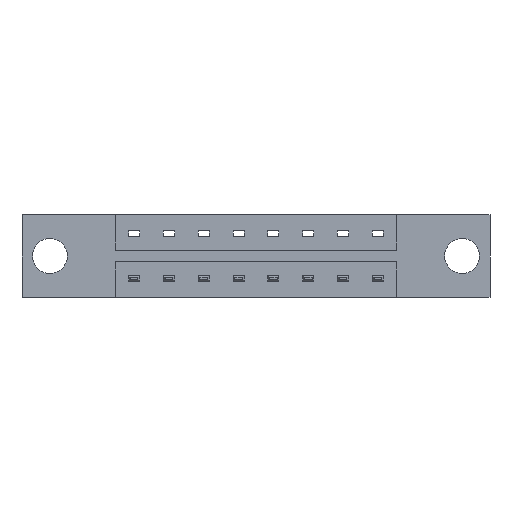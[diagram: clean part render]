
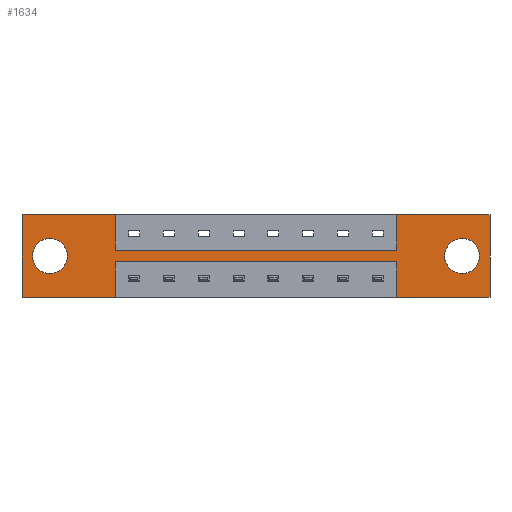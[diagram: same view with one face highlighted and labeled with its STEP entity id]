
A CAD part, front view. The second image highlights one B-rep face of the part: STEP entity #1634.
In plain terms, the highlighted planar face has unit normal (0, -1, 0).
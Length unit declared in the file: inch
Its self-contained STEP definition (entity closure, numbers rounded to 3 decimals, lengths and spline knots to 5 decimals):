
#97 = DIRECTION ( 'NONE',  ( 0., 0., -1. ) ) ;
#120 = PLANE ( 'NONE',  #6960 ) ;
#161 = ORIENTED_EDGE ( 'NONE', *, *, #1057, .F. ) ;
#222 = VERTEX_POINT ( 'NONE', #7036 ) ;
#249 = DIRECTION ( 'NONE',  ( 0., 1., 0. ) ) ;
#284 = DIRECTION ( 'NONE',  ( 0., 0., -1. ) ) ;
#331 = LINE ( 'NONE', #5976, #1162 ) ;
#354 = ORIENTED_EDGE ( 'NONE', *, *, #995, .F. ) ;
#361 = VECTOR ( 'NONE', #808, 39.37008 ) ;
#465 = CARTESIAN_POINT ( 'NONE',  ( 1.6785, 0., -0.2115 ) ) ;
#496 = EDGE_CURVE ( 'NONE', #8534, #3127, #938, .T. ) ;
#721 = VECTOR ( 'NONE', #1155, 39.37008 ) ;
#799 = VERTEX_POINT ( 'NONE', #5838 ) ;
#808 = DIRECTION ( 'NONE',  ( 0., 0., 1. ) ) ;
#862 = CARTESIAN_POINT ( 'NONE',  ( 2.096, 0., -0.37 ) ) ;
#866 = AXIS2_PLACEMENT_3D ( 'NONE', #2997, #7089, #2206 ) ;
#911 = FACE_OUTER_BOUND ( 'NONE', #1650, .T. ) ;
#921 = EDGE_CURVE ( 'NONE', #3524, #3013, #331, .T. ) ;
#938 = CIRCLE ( 'NONE', #2129, 0.078 ) ;
#964 = EDGE_LOOP ( 'NONE', ( #5237, #8915 ) ) ;
#995 = EDGE_CURVE ( 'NONE', #3325, #8049, #7485, .T. ) ;
#1000 = CARTESIAN_POINT ( 'NONE',  ( 1.6785, 0., -0.1585 ) ) ;
#1041 = CARTESIAN_POINT ( 'NONE',  ( 2.096, 0., 0. ) ) ;
#1057 = EDGE_CURVE ( 'NONE', #5483, #3524, #5420, .T. ) ;
#1097 = CARTESIAN_POINT ( 'NONE',  ( 0., 0., -0.37 ) ) ;
#1155 = DIRECTION ( 'NONE',  ( 0., 0., 1. ) ) ;
#1162 = VECTOR ( 'NONE', #284, 39.37008 ) ;
#1167 = ORIENTED_EDGE ( 'NONE', *, *, #3493, .F. ) ;
#1338 = LINE ( 'NONE', #5687, #8081 ) ;
#1478 = DIRECTION ( 'NONE',  ( -1., 0., 0. ) ) ;
#1533 = ORIENTED_EDGE ( 'NONE', *, *, #921, .F. ) ;
#1634 = ADVANCED_FACE ( 'NONE', ( #3048, #4310, #911 ), #120, .T. ) ;
#1635 = ORIENTED_EDGE ( 'NONE', *, *, #7399, .F. ) ;
#1650 = EDGE_LOOP ( 'NONE', ( #7386, #1805, #1533, #161, #2510, #6017, #1635, #354, #1167, #4787, #2770, #2639 ) ) ;
#1805 = ORIENTED_EDGE ( 'NONE', *, *, #3112, .F. ) ;
#1892 = VERTEX_POINT ( 'NONE', #5959 ) ;
#1901 = CARTESIAN_POINT ( 'NONE',  ( 0., 0., 0. ) ) ;
#2051 = CIRCLE ( 'NONE', #8232, 0.078 ) ;
#2129 = AXIS2_PLACEMENT_3D ( 'NONE', #6581, #249, #5895 ) ;
#2147 = EDGE_CURVE ( 'NONE', #3127, #8534, #3242, .T. ) ;
#2165 = VERTEX_POINT ( 'NONE', #4490 ) ;
#2206 = DIRECTION ( 'NONE',  ( 0., 0., 1. ) ) ;
#2250 = VERTEX_POINT ( 'NONE', #2610 ) ;
#2271 = DIRECTION ( 'NONE',  ( 0., 0., 1. ) ) ;
#2290 = DIRECTION ( 'NONE',  ( 0., 0., -1. ) ) ;
#2328 = VERTEX_POINT ( 'NONE', #4743 ) ;
#2404 = DIRECTION ( 'NONE',  ( 0., 0., -1. ) ) ;
#2406 = LINE ( 'NONE', #1000, #3681 ) ;
#2451 = LINE ( 'NONE', #5993, #9018 ) ;
#2510 = ORIENTED_EDGE ( 'NONE', *, *, #2916, .F. ) ;
#2610 = CARTESIAN_POINT ( 'NONE',  ( 1.6785, 0., -0.2115 ) ) ;
#2639 = ORIENTED_EDGE ( 'NONE', *, *, #4357, .F. ) ;
#2647 = VECTOR ( 'NONE', #8945, 39.37008 ) ;
#2770 = ORIENTED_EDGE ( 'NONE', *, *, #8570, .F. ) ;
#2815 = CARTESIAN_POINT ( 'NONE',  ( 0., 0., 0. ) ) ;
#2844 = AXIS2_PLACEMENT_3D ( 'NONE', #7637, #5534, #4193 ) ;
#2880 = EDGE_CURVE ( 'NONE', #2165, #799, #1338, .T. ) ;
#2916 = EDGE_CURVE ( 'NONE', #222, #5483, #2406, .T. ) ;
#2921 = EDGE_CURVE ( 'NONE', #5778, #1892, #2051, .T. ) ;
#2997 = CARTESIAN_POINT ( 'NONE',  ( 0.125, 0., -0.185 ) ) ;
#3013 = VERTEX_POINT ( 'NONE', #862 ) ;
#3048 = FACE_BOUND ( 'NONE', #4469, .T. ) ;
#3049 = DIRECTION ( 'NONE',  ( 0., 0., -1. ) ) ;
#3088 = DIRECTION ( 'NONE',  ( -1., 0., 0. ) ) ;
#3112 = EDGE_CURVE ( 'NONE', #3013, #8420, #3332, .T. ) ;
#3127 = VERTEX_POINT ( 'NONE', #3890 ) ;
#3242 = CIRCLE ( 'NONE', #866, 0.078 ) ;
#3279 = VECTOR ( 'NONE', #4741, 39.37008 ) ;
#3325 = VERTEX_POINT ( 'NONE', #2815 ) ;
#3332 = LINE ( 'NONE', #1097, #2647 ) ;
#3493 = EDGE_CURVE ( 'NONE', #799, #3325, #8708, .T. ) ;
#3524 = VERTEX_POINT ( 'NONE', #1041 ) ;
#3681 = VECTOR ( 'NONE', #2271, 39.37008 ) ;
#3714 = EDGE_CURVE ( 'NONE', #1892, #5778, #8430, .T. ) ;
#3810 = ORIENTED_EDGE ( 'NONE', *, *, #3714, .T. ) ;
#3843 = DIRECTION ( 'NONE',  ( 0., 1., 0. ) ) ;
#3890 = CARTESIAN_POINT ( 'NONE',  ( 0.125, 0., -0.107 ) ) ;
#4193 = DIRECTION ( 'NONE',  ( 0., 0., -1. ) ) ;
#4310 = FACE_BOUND ( 'NONE', #964, .T. ) ;
#4357 = EDGE_CURVE ( 'NONE', #2250, #7164, #2451, .T. ) ;
#4469 = EDGE_LOOP ( 'NONE', ( #3810, #5562 ) ) ;
#4490 = CARTESIAN_POINT ( 'NONE',  ( 0.4175, 0., -0.37 ) ) ;
#4614 = CARTESIAN_POINT ( 'NONE',  ( 0.4175, 0., -0.2115 ) ) ;
#4714 = EDGE_CURVE ( 'NONE', #2328, #222, #6488, .T. ) ;
#4741 = DIRECTION ( 'NONE',  ( 1., 0., 0. ) ) ;
#4743 = CARTESIAN_POINT ( 'NONE',  ( 0.4175, 0., -0.1585 ) ) ;
#4787 = ORIENTED_EDGE ( 'NONE', *, *, #2880, .F. ) ;
#4855 = VECTOR ( 'NONE', #8514, 39.37008 ) ;
#4871 = VECTOR ( 'NONE', #97, 39.37008 ) ;
#5237 = ORIENTED_EDGE ( 'NONE', *, *, #2147, .T. ) ;
#5420 = LINE ( 'NONE', #1901, #3279 ) ;
#5476 = VECTOR ( 'NONE', #2290, 39.37008 ) ;
#5483 = VERTEX_POINT ( 'NONE', #6736 ) ;
#5534 = DIRECTION ( 'NONE',  ( 0., 1., 0. ) ) ;
#5562 = ORIENTED_EDGE ( 'NONE', *, *, #2921, .T. ) ;
#5669 = CARTESIAN_POINT ( 'NONE',  ( 0.4175, 0., -0.1585 ) ) ;
#5687 = CARTESIAN_POINT ( 'NONE',  ( 0., 0., -0.37 ) ) ;
#5774 = DIRECTION ( 'NONE',  ( 0., -1., 0. ) ) ;
#5778 = VERTEX_POINT ( 'NONE', #6904 ) ;
#5838 = CARTESIAN_POINT ( 'NONE',  ( 0., 0., -0.37 ) ) ;
#5883 = LINE ( 'NONE', #4614, #5476 ) ;
#5895 = DIRECTION ( 'NONE',  ( 0., 0., 1. ) ) ;
#5959 = CARTESIAN_POINT ( 'NONE',  ( 1.971, 0., -0.107 ) ) ;
#5976 = CARTESIAN_POINT ( 'NONE',  ( 2.096, 0., 0. ) ) ;
#5993 = CARTESIAN_POINT ( 'NONE',  ( 0.4175, 0., -0.2115 ) ) ;
#6017 = ORIENTED_EDGE ( 'NONE', *, *, #4714, .F. ) ;
#6335 = LINE ( 'NONE', #6383, #4871 ) ;
#6383 = CARTESIAN_POINT ( 'NONE',  ( 0.4175, 0., -0.1585 ) ) ;
#6399 = CARTESIAN_POINT ( 'NONE',  ( 0., 0., 0. ) ) ;
#6488 = LINE ( 'NONE', #5669, #4855 ) ;
#6507 = VECTOR ( 'NONE', #7582, 39.37008 ) ;
#6581 = CARTESIAN_POINT ( 'NONE',  ( 0.125, 0., -0.185 ) ) ;
#6736 = CARTESIAN_POINT ( 'NONE',  ( 1.6785, 0., 0. ) ) ;
#6904 = CARTESIAN_POINT ( 'NONE',  ( 1.971, 0., -0.263 ) ) ;
#6960 = AXIS2_PLACEMENT_3D ( 'NONE', #8627, #5774, #2404 ) ;
#7036 = CARTESIAN_POINT ( 'NONE',  ( 1.6785, 0., -0.1585 ) ) ;
#7089 = DIRECTION ( 'NONE',  ( 0., 1., 0. ) ) ;
#7164 = VERTEX_POINT ( 'NONE', #7499 ) ;
#7386 = ORIENTED_EDGE ( 'NONE', *, *, #7587, .F. ) ;
#7399 = EDGE_CURVE ( 'NONE', #8049, #2328, #6335, .T. ) ;
#7485 = LINE ( 'NONE', #7535, #6507 ) ;
#7499 = CARTESIAN_POINT ( 'NONE',  ( 0.4175, 0., -0.2115 ) ) ;
#7535 = CARTESIAN_POINT ( 'NONE',  ( 0., 0., 0. ) ) ;
#7582 = DIRECTION ( 'NONE',  ( 1., 0., 0. ) ) ;
#7587 = EDGE_CURVE ( 'NONE', #8420, #2250, #9005, .T. ) ;
#7637 = CARTESIAN_POINT ( 'NONE',  ( 1.971, 0., -0.185 ) ) ;
#7823 = CARTESIAN_POINT ( 'NONE',  ( 0.125, 0., -0.263 ) ) ;
#7932 = CARTESIAN_POINT ( 'NONE',  ( 1.971, 0., -0.185 ) ) ;
#8049 = VERTEX_POINT ( 'NONE', #8128 ) ;
#8081 = VECTOR ( 'NONE', #1478, 39.37008 ) ;
#8128 = CARTESIAN_POINT ( 'NONE',  ( 0.4175, 0., 0. ) ) ;
#8232 = AXIS2_PLACEMENT_3D ( 'NONE', #7932, #3843, #3049 ) ;
#8420 = VERTEX_POINT ( 'NONE', #9019 ) ;
#8430 = CIRCLE ( 'NONE', #2844, 0.078 ) ;
#8514 = DIRECTION ( 'NONE',  ( 1., 0., 0. ) ) ;
#8534 = VERTEX_POINT ( 'NONE', #7823 ) ;
#8570 = EDGE_CURVE ( 'NONE', #7164, #2165, #5883, .T. ) ;
#8627 = CARTESIAN_POINT ( 'NONE',  ( 0., 0., -0.37 ) ) ;
#8708 = LINE ( 'NONE', #6399, #361 ) ;
#8915 = ORIENTED_EDGE ( 'NONE', *, *, #496, .T. ) ;
#8945 = DIRECTION ( 'NONE',  ( -1., 0., 0. ) ) ;
#9005 = LINE ( 'NONE', #465, #721 ) ;
#9018 = VECTOR ( 'NONE', #3088, 39.37008 ) ;
#9019 = CARTESIAN_POINT ( 'NONE',  ( 1.6785, 0., -0.37 ) ) ;
